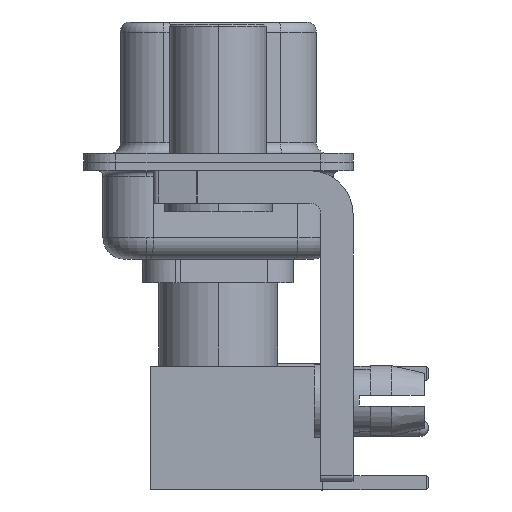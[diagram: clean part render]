
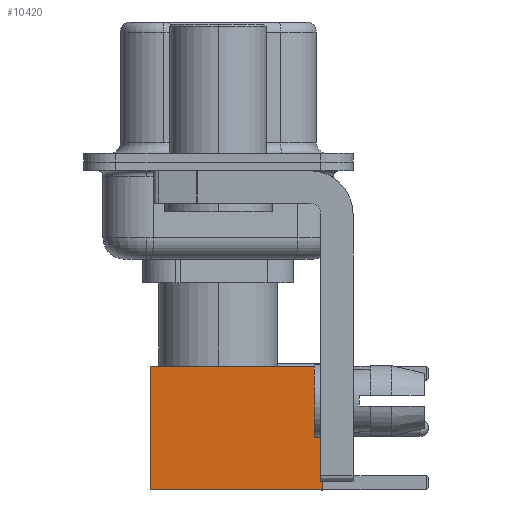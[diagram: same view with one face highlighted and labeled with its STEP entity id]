
A CAD part, left-side view. The second image highlights one B-rep face of the part: STEP entity #10420.
In plain terms, the highlighted face is planar.
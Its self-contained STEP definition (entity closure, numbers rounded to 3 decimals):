
#756 = DIRECTION ( 'NONE',  ( -1., 0., 0. ) ) ;
#1048 = CARTESIAN_POINT ( 'NONE',  ( -2.875, 2.875, 8. ) ) ;
#2969 = DIRECTION ( 'NONE',  ( 0., 0., 1. ) ) ;
#3010 = VECTOR ( 'NONE', #8380, 1000. ) ;
#3291 = VERTEX_POINT ( 'NONE', #17388 ) ;
#3789 = LINE ( 'NONE', #22768, #27594 ) ;
#5844 = PLANE ( 'NONE',  #19864 ) ;
#7482 = DIRECTION ( 'NONE',  ( 0., 0., -1. ) ) ;
#7517 = ORIENTED_EDGE ( 'NONE', *, *, #12005, .F. ) ;
#8274 = FACE_OUTER_BOUND ( 'NONE', #30626, .T. ) ;
#8380 = DIRECTION ( 'NONE',  ( 0., 0., -1. ) ) ;
#8843 = EDGE_CURVE ( 'NONE', #19944, #3291, #15042, .T. ) ;
#10332 = VECTOR ( 'NONE', #10458, 1000. ) ;
#10420 = ADVANCED_FACE ( 'NONE', ( #8274 ), #5844, .T. ) ;
#10458 = DIRECTION ( 'NONE',  ( -1., 0., 0. ) ) ;
#12005 = EDGE_CURVE ( 'NONE', #19944, #28191, #3789, .T. ) ;
#12867 = CARTESIAN_POINT ( 'NONE',  ( 0., 2.875, 0. ) ) ;
#13718 = ORIENTED_EDGE ( 'NONE', *, *, #22662, .T. ) ;
#15042 = LINE ( 'NONE', #30099, #28977 ) ;
#15199 = DIRECTION ( 'NONE',  ( 0., 1., 0. ) ) ;
#16156 = ORIENTED_EDGE ( 'NONE', *, *, #8843, .T. ) ;
#17388 = CARTESIAN_POINT ( 'NONE',  ( 2.875, 2.875, 0. ) ) ;
#18013 = LINE ( 'NONE', #12867, #10332 ) ;
#18085 = CARTESIAN_POINT ( 'NONE',  ( 2.875, 2.875, 0. ) ) ;
#19864 = AXIS2_PLACEMENT_3D ( 'NONE', #18085, #15199, #2969 ) ;
#19944 = VERTEX_POINT ( 'NONE', #20365 ) ;
#20040 = ORIENTED_EDGE ( 'NONE', *, *, #20773, .F. ) ;
#20293 = CARTESIAN_POINT ( 'NONE',  ( -2.875, 2.875, 0. ) ) ;
#20365 = CARTESIAN_POINT ( 'NONE',  ( 2.875, 2.875, 8. ) ) ;
#20773 = EDGE_CURVE ( 'NONE', #28191, #26113, #30372, .T. ) ;
#22597 = CARTESIAN_POINT ( 'NONE',  ( -2.875, 2.875, 0. ) ) ;
#22662 = EDGE_CURVE ( 'NONE', #3291, #26113, #18013, .T. ) ;
#22768 = CARTESIAN_POINT ( 'NONE',  ( 0., 2.875, 8. ) ) ;
#26113 = VERTEX_POINT ( 'NONE', #22597 ) ;
#27594 = VECTOR ( 'NONE', #756, 1000. ) ;
#28191 = VERTEX_POINT ( 'NONE', #1048 ) ;
#28977 = VECTOR ( 'NONE', #7482, 1000. ) ;
#30099 = CARTESIAN_POINT ( 'NONE',  ( 2.875, 2.875, 0. ) ) ;
#30372 = LINE ( 'NONE', #20293, #3010 ) ;
#30626 = EDGE_LOOP ( 'NONE', ( #16156, #13718, #20040, #7517 ) ) ;
